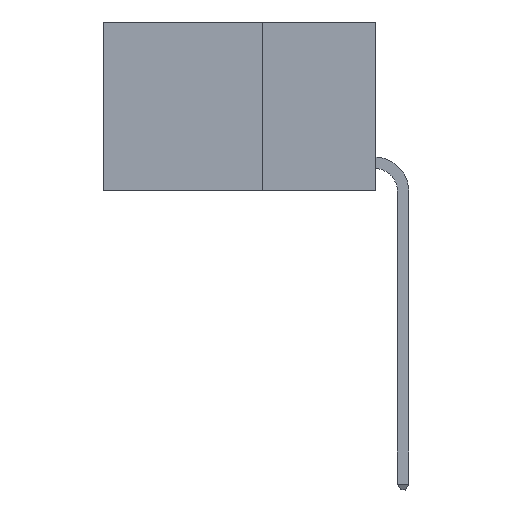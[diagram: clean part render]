
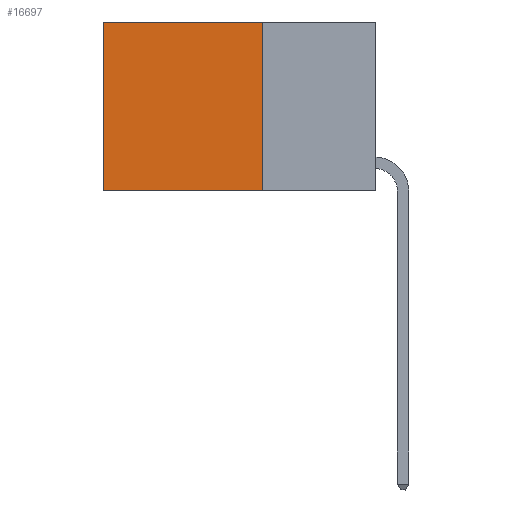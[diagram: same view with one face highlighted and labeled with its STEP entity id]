
A CAD part, left-side view. The second image highlights one B-rep face of the part: STEP entity #16697.
In plain terms, the highlighted planar face has unit normal (-1, 0, 0).
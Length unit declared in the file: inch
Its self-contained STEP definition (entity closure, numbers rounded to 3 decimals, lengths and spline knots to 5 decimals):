
#37 = DIRECTION ( 'NONE',  ( 0., 0., -1. ) ) ;
#496 = EDGE_CURVE ( 'NONE', #20870, #1022, #15488, .T. ) ;
#1022 = VERTEX_POINT ( 'NONE', #20583 ) ;
#1863 = CARTESIAN_POINT ( 'NONE',  ( 0.2625, 0.25, -0.37 ) ) ;
#2073 = FACE_OUTER_BOUND ( 'NONE', #15654, .T. ) ;
#2391 = LINE ( 'NONE', #16101, #16627 ) ;
#2601 = LINE ( 'NONE', #1863, #16826 ) ;
#3381 = CARTESIAN_POINT ( 'NONE',  ( 0.2625, 0.6, 0. ) ) ;
#4199 = EDGE_CURVE ( 'NONE', #20870, #15527, #2391, .T. ) ;
#5619 = VECTOR ( 'NONE', #23884, 39.37008 ) ;
#6110 = CARTESIAN_POINT ( 'NONE',  ( 0.2625, 0.25, 0. ) ) ;
#6537 = ORIENTED_EDGE ( 'NONE', *, *, #496, .F. ) ;
#7284 = VECTOR ( 'NONE', #18183, 39.37008 ) ;
#8779 = AXIS2_PLACEMENT_3D ( 'NONE', #22196, #11376, #37 ) ;
#8986 = EDGE_CURVE ( 'NONE', #15527, #16894, #12267, .T. ) ;
#9518 = PLANE ( 'NONE',  #8779 ) ;
#10673 = CARTESIAN_POINT ( 'NONE',  ( 0.2625, 0.6, 0. ) ) ;
#11376 = DIRECTION ( 'NONE',  ( 1., 0., 0. ) ) ;
#12267 = LINE ( 'NONE', #3381, #7284 ) ;
#12283 = ORIENTED_EDGE ( 'NONE', *, *, #8986, .T. ) ;
#13289 = CARTESIAN_POINT ( 'NONE',  ( 0.2625, 0.25, 0. ) ) ;
#15488 = LINE ( 'NONE', #6110, #5619 ) ;
#15527 = VERTEX_POINT ( 'NONE', #10673 ) ;
#15654 = EDGE_LOOP ( 'NONE', ( #12283, #21803, #6537, #19558 ) ) ;
#16101 = CARTESIAN_POINT ( 'NONE',  ( 0.2625, 0.25, 0. ) ) ;
#16627 = VECTOR ( 'NONE', #17891, 39.37008 ) ;
#16697 = ADVANCED_FACE ( 'NONE', ( #2073 ), #9518, .F. ) ;
#16826 = VECTOR ( 'NONE', #22136, 39.37008 ) ;
#16894 = VERTEX_POINT ( 'NONE', #19129 ) ;
#17891 = DIRECTION ( 'NONE',  ( 0., 1., 0. ) ) ;
#17960 = EDGE_CURVE ( 'NONE', #1022, #16894, #2601, .T. ) ;
#18183 = DIRECTION ( 'NONE',  ( 0., 0., -1. ) ) ;
#19129 = CARTESIAN_POINT ( 'NONE',  ( 0.2625, 0.6, -0.37 ) ) ;
#19558 = ORIENTED_EDGE ( 'NONE', *, *, #4199, .T. ) ;
#20583 = CARTESIAN_POINT ( 'NONE',  ( 0.2625, 0.25, -0.37 ) ) ;
#20870 = VERTEX_POINT ( 'NONE', #13289 ) ;
#21803 = ORIENTED_EDGE ( 'NONE', *, *, #17960, .F. ) ;
#22136 = DIRECTION ( 'NONE',  ( 0., 1., 0. ) ) ;
#22196 = CARTESIAN_POINT ( 'NONE',  ( 0.2625, 0.25, 0. ) ) ;
#23884 = DIRECTION ( 'NONE',  ( 0., 0., -1. ) ) ;
